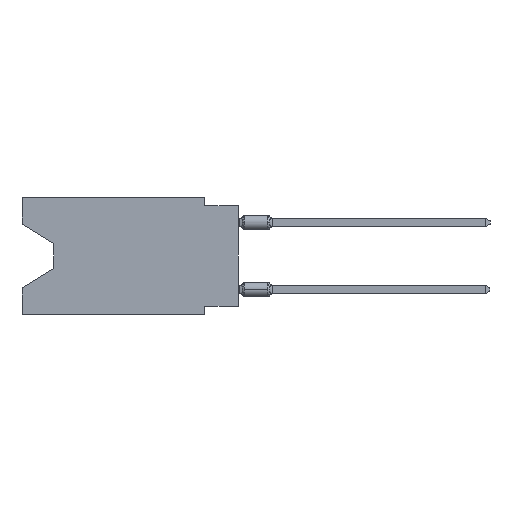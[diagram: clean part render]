
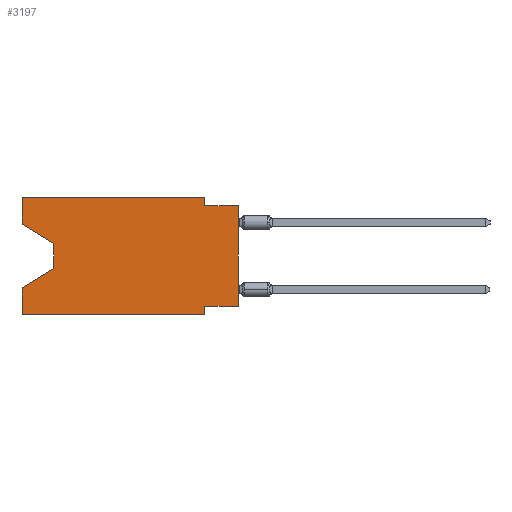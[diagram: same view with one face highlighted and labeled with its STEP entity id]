
A CAD part, left-side view. The second image highlights one B-rep face of the part: STEP entity #3197.
In plain terms, the highlighted planar face has unit normal (-1, 0, 0).
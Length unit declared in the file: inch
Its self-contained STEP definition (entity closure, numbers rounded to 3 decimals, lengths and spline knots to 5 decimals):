
#375 = ORIENTED_EDGE ( 'NONE', *, *, #42009, .F. ) ;
#391 = VERTEX_POINT ( 'NONE', #31663 ) ;
#670 = CARTESIAN_POINT ( 'NONE',  ( 0., 0., -0.025 ) ) ;
#736 = EDGE_CURVE ( 'NONE', #33474, #53909, #40612, .T. ) ;
#988 = VERTEX_POINT ( 'NONE', #29244 ) ;
#1668 = EDGE_CURVE ( 'NONE', #988, #21706, #59718, .T. ) ;
#2106 = VERTEX_POINT ( 'NONE', #38372 ) ;
#2226 = DIRECTION ( 'NONE',  ( 0., 0., -1. ) ) ;
#2438 = DIRECTION ( 'NONE',  ( 0., 0., 1. ) ) ;
#2582 = LINE ( 'NONE', #23523, #39722 ) ;
#3156 = LINE ( 'NONE', #54083, #37508 ) ;
#3197 = ADVANCED_FACE ( 'NONE', ( #31740 ), #21422, .F. ) ;
#3549 = CARTESIAN_POINT ( 'NONE',  ( 0., 0.55, -0.212 ) ) ;
#3772 = VERTEX_POINT ( 'NONE', #25099 ) ;
#3829 = CARTESIAN_POINT ( 'NONE',  ( 0., 0.645, 0. ) ) ;
#4469 = ORIENTED_EDGE ( 'NONE', *, *, #10307, .T. ) ;
#7435 = CARTESIAN_POINT ( 'NONE',  ( 0., 0.645, 0. ) ) ;
#7741 = EDGE_CURVE ( 'NONE', #64868, #3772, #50417, .T. ) ;
#8174 = CARTESIAN_POINT ( 'NONE',  ( 0., 0.645, 0. ) ) ;
#10307 = EDGE_CURVE ( 'NONE', #23452, #25144, #3156, .T. ) ;
#12420 = CARTESIAN_POINT ( 'NONE',  ( 0., 0.645, -0.08025 ) ) ;
#12551 = CARTESIAN_POINT ( 'NONE',  ( 0., 0.1, -0.35 ) ) ;
#12563 = DIRECTION ( 'NONE',  ( 0., 0.855, -0.519 ) ) ;
#12827 = VECTOR ( 'NONE', #49430, 39.37008 ) ;
#13679 = DIRECTION ( 'NONE',  ( 0., 1., 0. ) ) ;
#15152 = ORIENTED_EDGE ( 'NONE', *, *, #7741, .F. ) ;
#16118 = CARTESIAN_POINT ( 'NONE',  ( 0., 0.645, 0. ) ) ;
#16209 = EDGE_CURVE ( 'NONE', #988, #62632, #56208, .T. ) ;
#16890 = LINE ( 'NONE', #12551, #22328 ) ;
#17414 = EDGE_LOOP ( 'NONE', ( #24810, #4469, #29940, #33559, #43156, #51205, #46111, #45847, #27047, #375, #15152, #62071 ) ) ;
#18609 = CARTESIAN_POINT ( 'NONE',  ( 0., 0.55, -0.138 ) ) ;
#20442 = VECTOR ( 'NONE', #2438, 39.37008 ) ;
#21422 = PLANE ( 'NONE',  #33565 ) ;
#21436 = CARTESIAN_POINT ( 'NONE',  ( 0., 0.1, 0. ) ) ;
#21599 = VECTOR ( 'NONE', #64753, 39.37008 ) ;
#21706 = VERTEX_POINT ( 'NONE', #63761 ) ;
#22328 = VECTOR ( 'NONE', #2226, 39.37008 ) ;
#22406 = LINE ( 'NONE', #7435, #20442 ) ;
#22823 = VECTOR ( 'NONE', #51744, 39.37008 ) ;
#23008 = VECTOR ( 'NONE', #13679, 39.37008 ) ;
#23452 = VERTEX_POINT ( 'NONE', #18609 ) ;
#23523 = CARTESIAN_POINT ( 'NONE',  ( 0., 0.55, -0.212 ) ) ;
#24810 = ORIENTED_EDGE ( 'NONE', *, *, #59342, .T. ) ;
#25006 = EDGE_CURVE ( 'NONE', #2106, #62632, #16890, .T. ) ;
#25099 = CARTESIAN_POINT ( 'NONE',  ( 0., 0.1, 0. ) ) ;
#25144 = VERTEX_POINT ( 'NONE', #3549 ) ;
#27047 = ORIENTED_EDGE ( 'NONE', *, *, #736, .F. ) ;
#29244 = CARTESIAN_POINT ( 'NONE',  ( 0., 0.645, -0.35 ) ) ;
#29808 = CARTESIAN_POINT ( 'NONE',  ( 0., 0., 0. ) ) ;
#29940 = ORIENTED_EDGE ( 'NONE', *, *, #55021, .T. ) ;
#31663 = CARTESIAN_POINT ( 'NONE',  ( 0., 0., -0.325 ) ) ;
#31740 = FACE_OUTER_BOUND ( 'NONE', #17414, .T. ) ;
#33474 = VERTEX_POINT ( 'NONE', #49716 ) ;
#33559 = ORIENTED_EDGE ( 'NONE', *, *, #1668, .F. ) ;
#33565 = AXIS2_PLACEMENT_3D ( 'NONE', #16118, #36424, #52041 ) ;
#34767 = DIRECTION ( 'NONE',  ( 0., -1., 0. ) ) ;
#35480 = LINE ( 'NONE', #29808, #21599 ) ;
#36424 = DIRECTION ( 'NONE',  ( 1., 0., 0. ) ) ;
#36577 = CARTESIAN_POINT ( 'NONE',  ( 0., 0.1, -0.35 ) ) ;
#37349 = VECTOR ( 'NONE', #50225, 39.37008 ) ;
#37508 = VECTOR ( 'NONE', #63719, 39.37008 ) ;
#38021 = VECTOR ( 'NONE', #63322, 39.37008 ) ;
#38372 = CARTESIAN_POINT ( 'NONE',  ( 0., 0.1, -0.325 ) ) ;
#39722 = VECTOR ( 'NONE', #12563, 39.37008 ) ;
#40578 = CARTESIAN_POINT ( 'NONE',  ( 0., 0.645, -0.35 ) ) ;
#40612 = LINE ( 'NONE', #670, #63224 ) ;
#40731 = EDGE_CURVE ( 'NONE', #391, #53909, #35480, .T. ) ;
#42009 = EDGE_CURVE ( 'NONE', #3772, #33474, #65064, .T. ) ;
#43156 = ORIENTED_EDGE ( 'NONE', *, *, #16209, .T. ) ;
#43324 = CARTESIAN_POINT ( 'NONE',  ( 0., 0., -0.325 ) ) ;
#45793 = EDGE_CURVE ( 'NONE', #391, #2106, #48317, .T. ) ;
#45847 = ORIENTED_EDGE ( 'NONE', *, *, #40731, .T. ) ;
#46111 = ORIENTED_EDGE ( 'NONE', *, *, #45793, .F. ) ;
#48317 = LINE ( 'NONE', #43324, #23008 ) ;
#48369 = CARTESIAN_POINT ( 'NONE',  ( 0., 0.645, -0.08025 ) ) ;
#49430 = DIRECTION ( 'NONE',  ( 0., 0., 1. ) ) ;
#49716 = CARTESIAN_POINT ( 'NONE',  ( 0., 0.1, -0.025 ) ) ;
#50225 = DIRECTION ( 'NONE',  ( 0., -1., 0. ) ) ;
#50417 = LINE ( 'NONE', #55743, #55703 ) ;
#51205 = ORIENTED_EDGE ( 'NONE', *, *, #25006, .F. ) ;
#51256 = DIRECTION ( 'NONE',  ( 0., -1., 0. ) ) ;
#51744 = DIRECTION ( 'NONE',  ( 0., 0., -1. ) ) ;
#52041 = DIRECTION ( 'NONE',  ( 0., 0., -1. ) ) ;
#53909 = VERTEX_POINT ( 'NONE', #54792 ) ;
#54083 = CARTESIAN_POINT ( 'NONE',  ( 0., 0.55, -0.138 ) ) ;
#54792 = CARTESIAN_POINT ( 'NONE',  ( 0., 0., -0.025 ) ) ;
#55021 = EDGE_CURVE ( 'NONE', #25144, #21706, #2582, .T. ) ;
#55703 = VECTOR ( 'NONE', #34767, 39.37008 ) ;
#55743 = CARTESIAN_POINT ( 'NONE',  ( 0., 0.645, 0. ) ) ;
#56208 = LINE ( 'NONE', #40578, #37349 ) ;
#59342 = EDGE_CURVE ( 'NONE', #64712, #23452, #63644, .T. ) ;
#59718 = LINE ( 'NONE', #8174, #12827 ) ;
#60608 = EDGE_CURVE ( 'NONE', #64712, #64868, #22406, .T. ) ;
#62071 = ORIENTED_EDGE ( 'NONE', *, *, #60608, .F. ) ;
#62632 = VERTEX_POINT ( 'NONE', #36577 ) ;
#63224 = VECTOR ( 'NONE', #51256, 39.37008 ) ;
#63322 = DIRECTION ( 'NONE',  ( 0., -0.855, -0.519 ) ) ;
#63644 = LINE ( 'NONE', #48369, #38021 ) ;
#63719 = DIRECTION ( 'NONE',  ( 0., 0., -1. ) ) ;
#63761 = CARTESIAN_POINT ( 'NONE',  ( 0., 0.645, -0.26975 ) ) ;
#64712 = VERTEX_POINT ( 'NONE', #12420 ) ;
#64753 = DIRECTION ( 'NONE',  ( 0., 0., 1. ) ) ;
#64868 = VERTEX_POINT ( 'NONE', #3829 ) ;
#65064 = LINE ( 'NONE', #21436, #22823 ) ;
